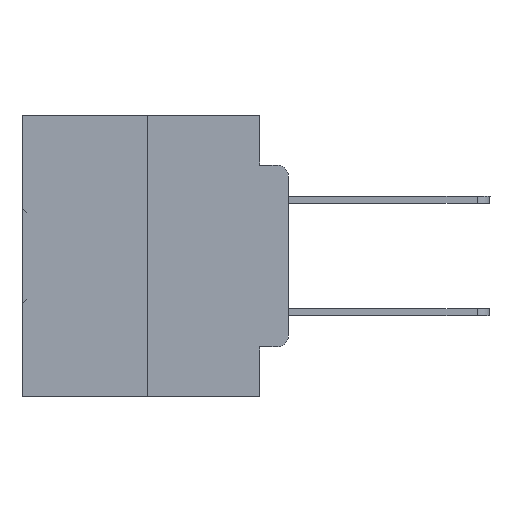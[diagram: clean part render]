
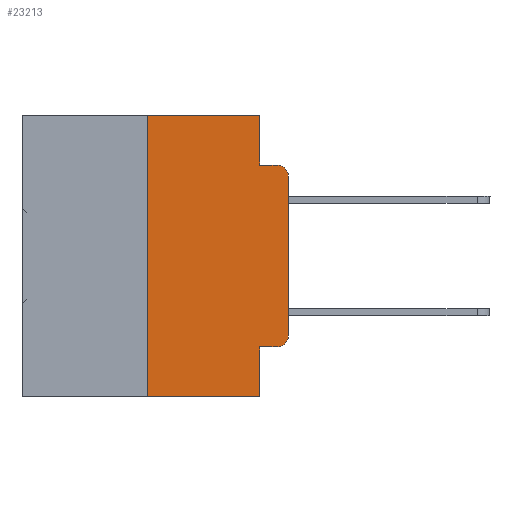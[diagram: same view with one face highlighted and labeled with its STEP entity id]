
A CAD part, left-side view. The second image highlights one B-rep face of the part: STEP entity #23213.
In plain terms, the highlighted planar face has unit normal (-1, 0, 0).
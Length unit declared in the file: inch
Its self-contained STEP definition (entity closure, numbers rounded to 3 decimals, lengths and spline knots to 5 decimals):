
#375 = VECTOR ( 'NONE', #17961, 39.37008 ) ;
#1235 = VERTEX_POINT ( 'NONE', #28912 ) ;
#1450 = ORIENTED_EDGE ( 'NONE', *, *, #8746, .F. ) ;
#1889 = LINE ( 'NONE', #18789, #16176 ) ;
#2062 = VERTEX_POINT ( 'NONE', #16674 ) ;
#3389 = CARTESIAN_POINT ( 'NONE',  ( 0., 0.051, -0.4115 ) ) ;
#4396 = LINE ( 'NONE', #28642, #5223 ) ;
#5100 = CARTESIAN_POINT ( 'NONE',  ( 0., 0.02, -0.3915 ) ) ;
#5213 = ORIENTED_EDGE ( 'NONE', *, *, #32782, .T. ) ;
#5223 = VECTOR ( 'NONE', #12872, 39.37008 ) ;
#5420 = DIRECTION ( 'NONE',  ( 0., -1., 0. ) ) ;
#5501 = DIRECTION ( 'NONE',  ( 1., 0., 0. ) ) ;
#5579 = CARTESIAN_POINT ( 'NONE',  ( 0., 0.25, 0. ) ) ;
#6056 = EDGE_LOOP ( 'NONE', ( #5213, #15854, #23210, #6880, #1450, #30440, #12098, #19523, #18272, #12441 ) ) ;
#6521 = AXIS2_PLACEMENT_3D ( 'NONE', #26892, #11026, #29486 ) ;
#6665 = DIRECTION ( 'NONE',  ( 0., -1., 0. ) ) ;
#6719 = VERTEX_POINT ( 'NONE', #3389 ) ;
#6880 = ORIENTED_EDGE ( 'NONE', *, *, #25843, .F. ) ;
#7465 = VECTOR ( 'NONE', #16749, 39.37008 ) ;
#7681 = CARTESIAN_POINT ( 'NONE',  ( 0., 0., -0.1085 ) ) ;
#7802 = DIRECTION ( 'NONE',  ( 0., 0., -1. ) ) ;
#8020 = VERTEX_POINT ( 'NONE', #16692 ) ;
#8746 = EDGE_CURVE ( 'NONE', #10231, #10386, #29614, .T. ) ;
#10231 = VERTEX_POINT ( 'NONE', #5579 ) ;
#10386 = VERTEX_POINT ( 'NONE', #19636 ) ;
#11026 = DIRECTION ( 'NONE',  ( -1., 0., 0. ) ) ;
#12098 = ORIENTED_EDGE ( 'NONE', *, *, #29778, .T. ) ;
#12441 = ORIENTED_EDGE ( 'NONE', *, *, #17023, .T. ) ;
#12872 = DIRECTION ( 'NONE',  ( 0., 0., -1. ) ) ;
#13123 = DIRECTION ( 'NONE',  ( 0., -1., 0. ) ) ;
#13597 = CIRCLE ( 'NONE', #25932, 0.02 ) ;
#13819 = LINE ( 'NONE', #33618, #375 ) ;
#14619 = DIRECTION ( 'NONE',  ( 0., 0., -1. ) ) ;
#15191 = VERTEX_POINT ( 'NONE', #29354 ) ;
#15484 = LINE ( 'NONE', #29819, #7465 ) ;
#15854 = ORIENTED_EDGE ( 'NONE', *, *, #29327, .T. ) ;
#16176 = VECTOR ( 'NONE', #5420, 39.37008 ) ;
#16353 = CARTESIAN_POINT ( 'NONE',  ( 0., 0., 0. ) ) ;
#16384 = VECTOR ( 'NONE', #32138, 39.37008 ) ;
#16674 = CARTESIAN_POINT ( 'NONE',  ( 0., 0.051, -0.5 ) ) ;
#16692 = CARTESIAN_POINT ( 'NONE',  ( 0., 0.02, -0.0885 ) ) ;
#16749 = DIRECTION ( 'NONE',  ( 0., -1., 0. ) ) ;
#17023 = EDGE_CURVE ( 'NONE', #18980, #18135, #13597, .T. ) ;
#17357 = CARTESIAN_POINT ( 'NONE',  ( 0., 0.051, -0.4115 ) ) ;
#17961 = DIRECTION ( 'NONE',  ( 0., 0., 1. ) ) ;
#18135 = VERTEX_POINT ( 'NONE', #33064 ) ;
#18272 = ORIENTED_EDGE ( 'NONE', *, *, #18782, .T. ) ;
#18782 = EDGE_CURVE ( 'NONE', #6719, #18980, #27505, .T. ) ;
#18789 = CARTESIAN_POINT ( 'NONE',  ( 0., 0.473, -0.5 ) ) ;
#18865 = CARTESIAN_POINT ( 'NONE',  ( 0., 0.473, 0. ) ) ;
#18980 = VERTEX_POINT ( 'NONE', #21285 ) ;
#19523 = ORIENTED_EDGE ( 'NONE', *, *, #20544, .F. ) ;
#19636 = CARTESIAN_POINT ( 'NONE',  ( 0., 0.051, 0. ) ) ;
#19922 = VECTOR ( 'NONE', #14619, 39.37008 ) ;
#20514 = VECTOR ( 'NONE', #6665, 39.37008 ) ;
#20544 = EDGE_CURVE ( 'NONE', #6719, #2062, #4396, .T. ) ;
#21285 = CARTESIAN_POINT ( 'NONE',  ( 0., 0.02, -0.4115 ) ) ;
#23210 = ORIENTED_EDGE ( 'NONE', *, *, #27595, .F. ) ;
#23213 = ADVANCED_FACE ( 'NONE', ( #32349 ), #31889, .F. ) ;
#23220 = CIRCLE ( 'NONE', #6521, 0.02 ) ;
#23397 = AXIS2_PLACEMENT_3D ( 'NONE', #18865, #5501, #24166 ) ;
#23536 = VERTEX_POINT ( 'NONE', #7681 ) ;
#23766 = DIRECTION ( 'NONE',  ( -1., 0., 0. ) ) ;
#24078 = EDGE_CURVE ( 'NONE', #15191, #10231, #13819, .T. ) ;
#24166 = DIRECTION ( 'NONE',  ( 0., 0., -1. ) ) ;
#25843 = EDGE_CURVE ( 'NONE', #10386, #1235, #27725, .T. ) ;
#25932 = AXIS2_PLACEMENT_3D ( 'NONE', #5100, #23766, #7802 ) ;
#26291 = CARTESIAN_POINT ( 'NONE',  ( 0., 0.473, 0. ) ) ;
#26892 = CARTESIAN_POINT ( 'NONE',  ( 0., 0.02, -0.1085 ) ) ;
#27505 = LINE ( 'NONE', #17357, #20514 ) ;
#27595 = EDGE_CURVE ( 'NONE', #1235, #8020, #15484, .T. ) ;
#27725 = LINE ( 'NONE', #32964, #19922 ) ;
#28642 = CARTESIAN_POINT ( 'NONE',  ( 0., 0.051, 0. ) ) ;
#28787 = VECTOR ( 'NONE', #13123, 39.37008 ) ;
#28912 = CARTESIAN_POINT ( 'NONE',  ( 0., 0.051, -0.0885 ) ) ;
#29327 = EDGE_CURVE ( 'NONE', #23536, #8020, #23220, .T. ) ;
#29354 = CARTESIAN_POINT ( 'NONE',  ( 0., 0.25, -0.5 ) ) ;
#29486 = DIRECTION ( 'NONE',  ( 0., 0., -1. ) ) ;
#29614 = LINE ( 'NONE', #26291, #28787 ) ;
#29778 = EDGE_CURVE ( 'NONE', #15191, #2062, #1889, .T. ) ;
#29819 = CARTESIAN_POINT ( 'NONE',  ( 0., 0.051, -0.0885 ) ) ;
#30321 = LINE ( 'NONE', #16353, #16384 ) ;
#30440 = ORIENTED_EDGE ( 'NONE', *, *, #24078, .F. ) ;
#31889 = PLANE ( 'NONE',  #23397 ) ;
#32138 = DIRECTION ( 'NONE',  ( 0., 0., 1. ) ) ;
#32349 = FACE_OUTER_BOUND ( 'NONE', #6056, .T. ) ;
#32782 = EDGE_CURVE ( 'NONE', #18135, #23536, #30321, .T. ) ;
#32964 = CARTESIAN_POINT ( 'NONE',  ( 0., 0.051, 0. ) ) ;
#33064 = CARTESIAN_POINT ( 'NONE',  ( 0., 0., -0.3915 ) ) ;
#33618 = CARTESIAN_POINT ( 'NONE',  ( 0., 0.25, 0. ) ) ;
